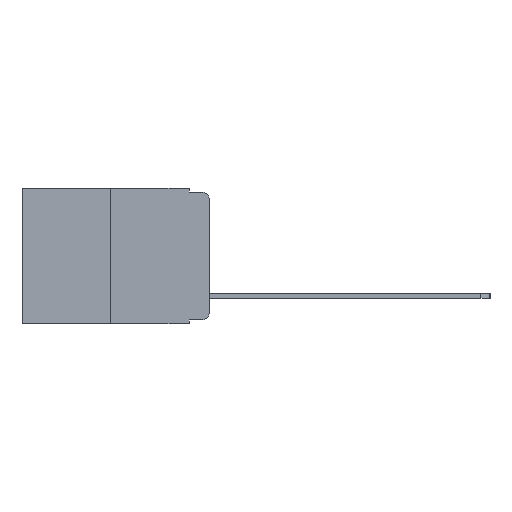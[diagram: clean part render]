
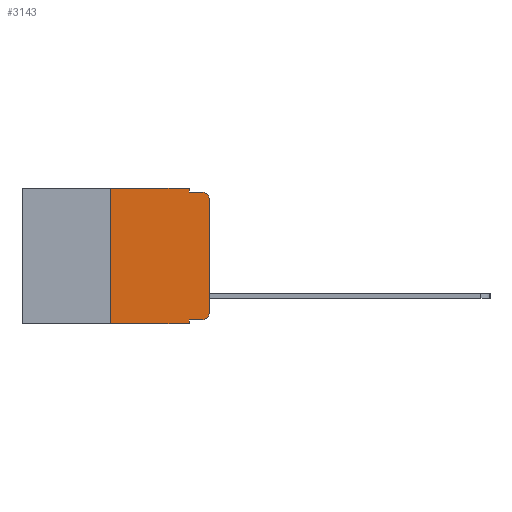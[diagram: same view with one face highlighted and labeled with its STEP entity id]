
A CAD part, left-side view. The second image highlights one B-rep face of the part: STEP entity #3143.
In plain terms, the highlighted planar face has unit normal (-1, 0, 0).
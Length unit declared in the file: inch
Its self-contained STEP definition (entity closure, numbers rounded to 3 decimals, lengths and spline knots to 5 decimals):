
#19 = DIRECTION ( 'NONE',  ( 0., -1., 0. ) ) ;
#98 = EDGE_CURVE ( 'NONE', #6440, #2710, #7797, .T. ) ;
#418 = LINE ( 'NONE', #4629, #5453 ) ;
#434 = EDGE_CURVE ( 'NONE', #3315, #11280, #418, .T. ) ;
#708 = EDGE_CURVE ( 'NONE', #2710, #7959, #7786, .T. ) ;
#963 = DIRECTION ( 'NONE',  ( 0., -1., 0. ) ) ;
#972 = VECTOR ( 'NONE', #963, 39.37008 ) ;
#1154 = VERTEX_POINT ( 'NONE', #4496 ) ;
#1389 = DIRECTION ( 'NONE',  ( 0., 0., 1. ) ) ;
#1615 = CIRCLE ( 'NONE', #5864, 0.02 ) ;
#1655 = CARTESIAN_POINT ( 'NONE',  ( 0., 0.25, 0. ) ) ;
#1843 = DIRECTION ( 'NONE',  ( 0., 0., -1. ) ) ;
#1863 = DIRECTION ( 'NONE',  ( 1., 0., 0. ) ) ;
#1904 = PLANE ( 'NONE',  #8449 ) ;
#1929 = VECTOR ( 'NONE', #19, 39.37008 ) ;
#1963 = CARTESIAN_POINT ( 'NONE',  ( 0., 0.02, -0.313 ) ) ;
#1994 = CARTESIAN_POINT ( 'NONE',  ( 0., 0.473, 0. ) ) ;
#2262 = VERTEX_POINT ( 'NONE', #6500 ) ;
#2310 = VERTEX_POINT ( 'NONE', #4398 ) ;
#2702 = CARTESIAN_POINT ( 'NONE',  ( 0., 0.25, -0.343 ) ) ;
#2710 = VERTEX_POINT ( 'NONE', #10761 ) ;
#2774 = EDGE_CURVE ( 'NONE', #2262, #7959, #5114, .T. ) ;
#2859 = DIRECTION ( 'NONE',  ( 0., 0., -1. ) ) ;
#3064 = DIRECTION ( 'NONE',  ( 0., 0., -1. ) ) ;
#3118 = CARTESIAN_POINT ( 'NONE',  ( 0., 0.051, 0. ) ) ;
#3143 = ADVANCED_FACE ( 'NONE', ( #6059 ), #1904, .F. ) ;
#3294 = VECTOR ( 'NONE', #1389, 39.37008 ) ;
#3315 = VERTEX_POINT ( 'NONE', #2702 ) ;
#3438 = EDGE_LOOP ( 'NONE', ( #4335, #4450, #4494, #4694, #4778, #4790, #4977, #4821, #5001, #5073 ) ) ;
#3661 = VECTOR ( 'NONE', #2859, 39.37008 ) ;
#3728 = CARTESIAN_POINT ( 'NONE',  ( 0., 0.051, -0.333 ) ) ;
#3785 = LINE ( 'NONE', #6810, #972 ) ;
#4190 = CARTESIAN_POINT ( 'NONE',  ( 0., 0.02, -0.03 ) ) ;
#4335 = ORIENTED_EDGE ( 'NONE', *, *, #6603, .T. ) ;
#4398 = CARTESIAN_POINT ( 'NONE',  ( 0., 0., -0.313 ) ) ;
#4450 = ORIENTED_EDGE ( 'NONE', *, *, #2774, .T. ) ;
#4494 = ORIENTED_EDGE ( 'NONE', *, *, #708, .F. ) ;
#4496 = CARTESIAN_POINT ( 'NONE',  ( 0., 0.25, 0. ) ) ;
#4515 = CARTESIAN_POINT ( 'NONE',  ( 0., 0., 0. ) ) ;
#4629 = CARTESIAN_POINT ( 'NONE',  ( 0., 0.473, -0.343 ) ) ;
#4694 = ORIENTED_EDGE ( 'NONE', *, *, #98, .F. ) ;
#4778 = ORIENTED_EDGE ( 'NONE', *, *, #6872, .F. ) ;
#4790 = ORIENTED_EDGE ( 'NONE', *, *, #9903, .F. ) ;
#4821 = ORIENTED_EDGE ( 'NONE', *, *, #8918, .F. ) ;
#4853 = AXIS2_PLACEMENT_3D ( 'NONE', #4190, #6240, #6151 ) ;
#4977 = ORIENTED_EDGE ( 'NONE', *, *, #434, .T. ) ;
#5001 = ORIENTED_EDGE ( 'NONE', *, *, #8391, .T. ) ;
#5016 = LINE ( 'NONE', #9561, #6776 ) ;
#5073 = ORIENTED_EDGE ( 'NONE', *, *, #6257, .T. ) ;
#5114 = CIRCLE ( 'NONE', #4853, 0.02 ) ;
#5453 = VECTOR ( 'NONE', #11242, 39.37008 ) ;
#5851 = LINE ( 'NONE', #4515, #3294 ) ;
#5864 = AXIS2_PLACEMENT_3D ( 'NONE', #1963, #8371, #3064 ) ;
#5932 = VERTEX_POINT ( 'NONE', #3728 ) ;
#6059 = FACE_OUTER_BOUND ( 'NONE', #3438, .T. ) ;
#6122 = VECTOR ( 'NONE', #8043, 39.37008 ) ;
#6151 = DIRECTION ( 'NONE',  ( 0., 0., -1. ) ) ;
#6240 = DIRECTION ( 'NONE',  ( -1., 0., 0. ) ) ;
#6257 = EDGE_CURVE ( 'NONE', #7466, #2310, #1615, .T. ) ;
#6440 = VERTEX_POINT ( 'NONE', #7766 ) ;
#6500 = CARTESIAN_POINT ( 'NONE',  ( 0., 0., -0.03 ) ) ;
#6603 = EDGE_CURVE ( 'NONE', #2310, #2262, #5851, .T. ) ;
#6776 = VECTOR ( 'NONE', #11078, 39.37008 ) ;
#6786 = CARTESIAN_POINT ( 'NONE',  ( 0., 0.051, -0.333 ) ) ;
#6810 = CARTESIAN_POINT ( 'NONE',  ( 0., 0.473, 0. ) ) ;
#6872 = EDGE_CURVE ( 'NONE', #1154, #6440, #3785, .T. ) ;
#6916 = LINE ( 'NONE', #1655, #10744 ) ;
#7057 = LINE ( 'NONE', #6786, #1929 ) ;
#7346 = CARTESIAN_POINT ( 'NONE',  ( 0., 0.051, -0.343 ) ) ;
#7466 = VERTEX_POINT ( 'NONE', #8308 ) ;
#7766 = CARTESIAN_POINT ( 'NONE',  ( 0., 0.051, 0. ) ) ;
#7786 = LINE ( 'NONE', #8775, #6122 ) ;
#7797 = LINE ( 'NONE', #3118, #3661 ) ;
#7959 = VERTEX_POINT ( 'NONE', #9511 ) ;
#8043 = DIRECTION ( 'NONE',  ( 0., -1., 0. ) ) ;
#8308 = CARTESIAN_POINT ( 'NONE',  ( 0., 0.02, -0.333 ) ) ;
#8371 = DIRECTION ( 'NONE',  ( -1., 0., 0. ) ) ;
#8391 = EDGE_CURVE ( 'NONE', #5932, #7466, #7057, .T. ) ;
#8449 = AXIS2_PLACEMENT_3D ( 'NONE', #1994, #1863, #1843 ) ;
#8775 = CARTESIAN_POINT ( 'NONE',  ( 0., 0.051, -0.01 ) ) ;
#8918 = EDGE_CURVE ( 'NONE', #5932, #11280, #5016, .T. ) ;
#9511 = CARTESIAN_POINT ( 'NONE',  ( 0., 0.02, -0.01 ) ) ;
#9561 = CARTESIAN_POINT ( 'NONE',  ( 0., 0.051, 0. ) ) ;
#9663 = DIRECTION ( 'NONE',  ( 0., 0., 1. ) ) ;
#9903 = EDGE_CURVE ( 'NONE', #3315, #1154, #6916, .T. ) ;
#10744 = VECTOR ( 'NONE', #9663, 39.37008 ) ;
#10761 = CARTESIAN_POINT ( 'NONE',  ( 0., 0.051, -0.01 ) ) ;
#11078 = DIRECTION ( 'NONE',  ( 0., 0., -1. ) ) ;
#11242 = DIRECTION ( 'NONE',  ( 0., -1., 0. ) ) ;
#11280 = VERTEX_POINT ( 'NONE', #7346 ) ;
